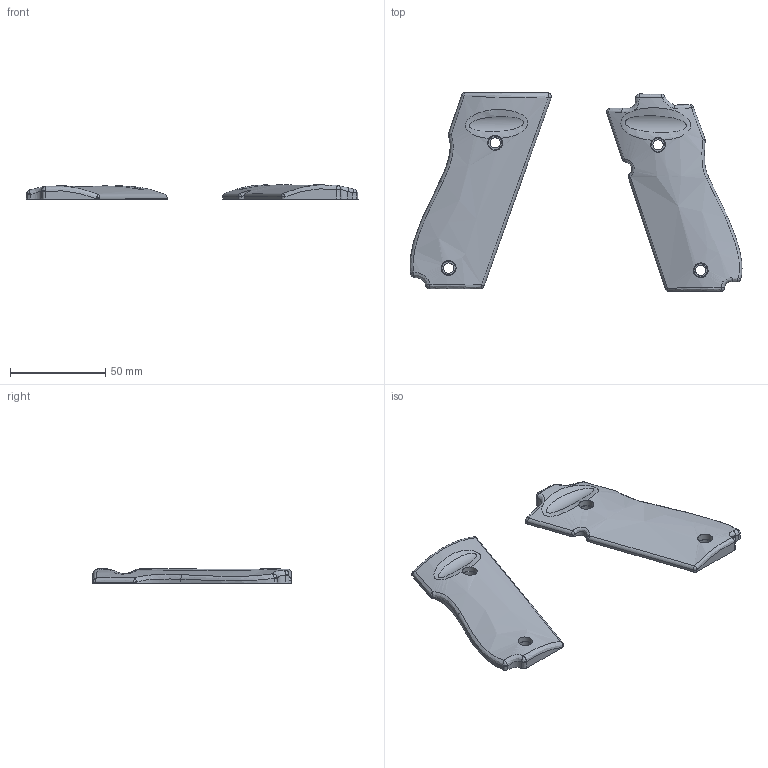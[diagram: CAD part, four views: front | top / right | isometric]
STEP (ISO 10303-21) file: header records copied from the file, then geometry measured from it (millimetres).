
FILE_DESCRIPTION(/* description */ (''),/* implementation_level */ '2;1');
FILE_NAME(/* name */ 'Grips v9.step',/* time_stamp */ '2020-04-11T04:46:58-04:00',/* author */ (''),/* organization */ (''),/* preprocessor_version */ 'ST-DEVELOPER v18',/* originating_system */ 'Autodesk Translation Framework v8.12.0.6',/* authorisation */ '');
FILE_SCHEMA (('AUTOMOTIVE_DESIGN { 1 0 10303 214 3 1 1 }'));
Length unit declared in the file: millimetre
Products named in the file (1): Grips
Bounding box: 174.23 x 104.38 x 7.46 mm (x, y, z)
Volume: 48409.1 mm3; surface area: 20435.8 mm2
Topology: 2 solids, 2 shells, 117 faces, 284 edges, 172 vertices
Faces by surface type: bspline 53, plane 29, cylinder 25, sphere 10
Full cylindrical faces by diameter (mm): 5.381 x4, 7 x4, 7.75 x4
Entity records: 5346 total; most frequent: CARTESIAN_POINT 2982, ORIENTED_EDGE 556, DIRECTION 345, EDGE_CURVE 278, VERTEX_POINT 172, AXIS2_PLACEMENT_3D 140, B_SPLINE_CURVE_WITH_KNOTS 135, EDGE_LOOP 132
